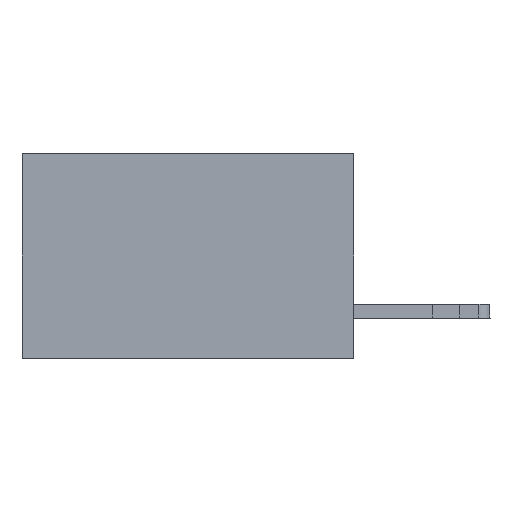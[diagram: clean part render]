
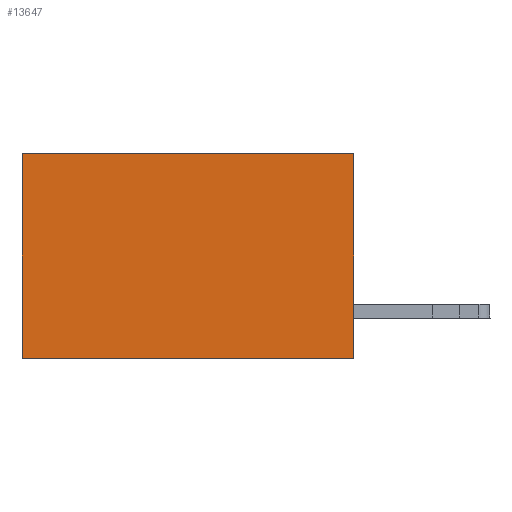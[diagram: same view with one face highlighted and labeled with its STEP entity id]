
A CAD part, left-side view. The second image highlights one B-rep face of the part: STEP entity #13647.
In plain terms, the highlighted planar face has unit normal (-1, 0, 0).
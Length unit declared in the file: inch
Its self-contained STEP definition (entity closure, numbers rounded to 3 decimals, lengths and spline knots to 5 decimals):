
#600 = CARTESIAN_POINT ( 'NONE',  ( 0.2875, 0., 0. ) ) ;
#2424 = DIRECTION ( 'NONE',  ( 1., 0., 0. ) ) ;
#2446 = DIRECTION ( 'NONE',  ( 0., 0., -1. ) ) ;
#3071 = VECTOR ( 'NONE', #20648, 39.37008 ) ;
#3639 = ORIENTED_EDGE ( 'NONE', *, *, #16271, .T. ) ;
#3751 = VERTEX_POINT ( 'NONE', #20795 ) ;
#3922 = VERTEX_POINT ( 'NONE', #10438 ) ;
#4505 = VERTEX_POINT ( 'NONE', #13920 ) ;
#4720 = PLANE ( 'NONE',  #24031 ) ;
#4933 = EDGE_CURVE ( 'NONE', #3922, #3751, #8641, .T. ) ;
#6252 = VECTOR ( 'NONE', #15501, 39.37008 ) ;
#6738 = CARTESIAN_POINT ( 'NONE',  ( 0.2875, 0.6, 0. ) ) ;
#7080 = CARTESIAN_POINT ( 'NONE',  ( 0.2875, 0.6, 0. ) ) ;
#8641 = LINE ( 'NONE', #25878, #6252 ) ;
#8849 = LINE ( 'NONE', #600, #3071 ) ;
#9878 = DIRECTION ( 'NONE',  ( 0., 0., -1. ) ) ;
#10438 = CARTESIAN_POINT ( 'NONE',  ( 0.2875, 0., -0.37 ) ) ;
#11469 = DIRECTION ( 'NONE',  ( 0., 0., -1. ) ) ;
#11982 = LINE ( 'NONE', #6738, #22510 ) ;
#13596 = EDGE_LOOP ( 'NONE', ( #19884, #19015, #17293, #3639 ) ) ;
#13647 = ADVANCED_FACE ( 'NONE', ( #18543 ), #4720, .F. ) ;
#13920 = CARTESIAN_POINT ( 'NONE',  ( 0.2875, 0., 0. ) ) ;
#15501 = DIRECTION ( 'NONE',  ( 0., 1., 0. ) ) ;
#16271 = EDGE_CURVE ( 'NONE', #4505, #24550, #8849, .T. ) ;
#17293 = ORIENTED_EDGE ( 'NONE', *, *, #24653, .F. ) ;
#17671 = VECTOR ( 'NONE', #9878, 39.37008 ) ;
#18543 = FACE_OUTER_BOUND ( 'NONE', #13596, .T. ) ;
#18837 = CARTESIAN_POINT ( 'NONE',  ( 0.2875, 0., 0. ) ) ;
#19015 = ORIENTED_EDGE ( 'NONE', *, *, #4933, .F. ) ;
#19884 = ORIENTED_EDGE ( 'NONE', *, *, #23353, .T. ) ;
#20648 = DIRECTION ( 'NONE',  ( 0., 1., 0. ) ) ;
#20795 = CARTESIAN_POINT ( 'NONE',  ( 0.2875, 0.6, -0.37 ) ) ;
#22274 = CARTESIAN_POINT ( 'NONE',  ( 0.2875, 0., 0. ) ) ;
#22510 = VECTOR ( 'NONE', #2446, 39.37008 ) ;
#23353 = EDGE_CURVE ( 'NONE', #24550, #3751, #11982, .T. ) ;
#23768 = LINE ( 'NONE', #18837, #17671 ) ;
#24031 = AXIS2_PLACEMENT_3D ( 'NONE', #22274, #2424, #11469 ) ;
#24550 = VERTEX_POINT ( 'NONE', #7080 ) ;
#24653 = EDGE_CURVE ( 'NONE', #4505, #3922, #23768, .T. ) ;
#25878 = CARTESIAN_POINT ( 'NONE',  ( 0.2875, 0., -0.37 ) ) ;
